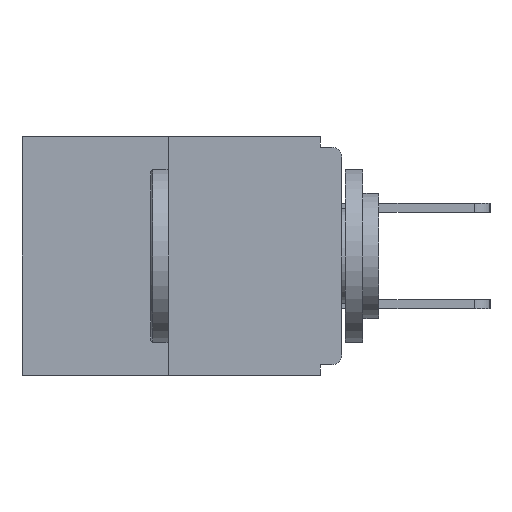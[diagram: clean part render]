
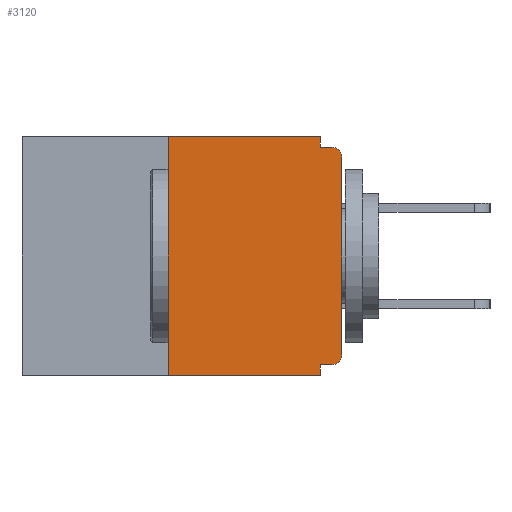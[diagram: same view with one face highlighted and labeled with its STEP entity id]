
A CAD part, left-side view. The second image highlights one B-rep face of the part: STEP entity #3120.
In plain terms, the highlighted planar face has unit normal (-1, 0, 0).
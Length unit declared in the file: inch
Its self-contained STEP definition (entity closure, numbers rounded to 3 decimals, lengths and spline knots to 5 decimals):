
#136 = DIRECTION ( 'NONE',  ( -1., 0., 0. ) ) ;
#253 = DIRECTION ( 'NONE',  ( 0., 0., -1. ) ) ;
#395 = ORIENTED_EDGE ( 'NONE', *, *, #1870, .T. ) ;
#508 = DIRECTION ( 'NONE',  ( 0., 0., 1. ) ) ;
#666 = ORIENTED_EDGE ( 'NONE', *, *, #10971, .F. ) ;
#798 = DIRECTION ( 'NONE',  ( 0., -1., 0. ) ) ;
#856 = LINE ( 'NONE', #7410, #12276 ) ;
#897 = ORIENTED_EDGE ( 'NONE', *, *, #1680, .F. ) ;
#1203 = DIRECTION ( 'NONE',  ( 0., 0., -1. ) ) ;
#1207 = VERTEX_POINT ( 'NONE', #2862 ) ;
#1286 = VERTEX_POINT ( 'NONE', #4184 ) ;
#1444 = AXIS2_PLACEMENT_3D ( 'NONE', #9204, #136, #1203 ) ;
#1544 = CARTESIAN_POINT ( 'NONE',  ( 0., 0., -0.313 ) ) ;
#1654 = LINE ( 'NONE', #8985, #3957 ) ;
#1680 = EDGE_CURVE ( 'NONE', #10077, #8715, #10153, .T. ) ;
#1840 = EDGE_CURVE ( 'NONE', #1286, #8715, #12437, .T. ) ;
#1843 = DIRECTION ( 'NONE',  ( 0., 0., 1. ) ) ;
#1870 = EDGE_CURVE ( 'NONE', #4796, #1286, #8736, .T. ) ;
#2024 = EDGE_CURVE ( 'NONE', #9354, #7687, #9660, .T. ) ;
#2215 = CARTESIAN_POINT ( 'NONE',  ( 0., 0.031, 0. ) ) ;
#2283 = EDGE_CURVE ( 'NONE', #7687, #10648, #856, .T. ) ;
#2366 = DIRECTION ( 'NONE',  ( 0., -1., 0. ) ) ;
#2507 = AXIS2_PLACEMENT_3D ( 'NONE', #6550, #2586, #12384 ) ;
#2586 = DIRECTION ( 'NONE',  ( 1., 0., 0. ) ) ;
#2814 = ORIENTED_EDGE ( 'NONE', *, *, #11748, .F. ) ;
#2862 = CARTESIAN_POINT ( 'NONE',  ( 0., 0.031, -0.343 ) ) ;
#2890 = CARTESIAN_POINT ( 'NONE',  ( 0., 0.25, 0. ) ) ;
#3120 = ADVANCED_FACE ( 'NONE', ( #11782 ), #4464, .F. ) ;
#3428 = EDGE_CURVE ( 'NONE', #9354, #1207, #8566, .T. ) ;
#3470 = EDGE_CURVE ( 'NONE', #10443, #4796, #7802, .T. ) ;
#3684 = CARTESIAN_POINT ( 'NONE',  ( 0., 0., -0.015 ) ) ;
#3781 = CARTESIAN_POINT ( 'NONE',  ( 0., 0.25, -0.343 ) ) ;
#3923 = ORIENTED_EDGE ( 'NONE', *, *, #1840, .T. ) ;
#3928 = CARTESIAN_POINT ( 'NONE',  ( 0., 0.031, -0.343 ) ) ;
#3957 = VECTOR ( 'NONE', #9028, 39.37008 ) ;
#4184 = CARTESIAN_POINT ( 'NONE',  ( 0., 0., -0.03 ) ) ;
#4430 = DIRECTION ( 'NONE',  ( 0., 0., -1. ) ) ;
#4464 = PLANE ( 'NONE',  #2507 ) ;
#4641 = EDGE_LOOP ( 'NONE', ( #4935, #12086, #10550, #8387, #666, #7011, #395, #3923, #897, #2814 ) ) ;
#4671 = CARTESIAN_POINT ( 'NONE',  ( 0., 0.031, -0.015 ) ) ;
#4796 = VERTEX_POINT ( 'NONE', #1544 ) ;
#4822 = LINE ( 'NONE', #3928, #5462 ) ;
#4935 = ORIENTED_EDGE ( 'NONE', *, *, #2283, .F. ) ;
#5242 = CARTESIAN_POINT ( 'NONE',  ( 0., 0., 0. ) ) ;
#5258 = AXIS2_PLACEMENT_3D ( 'NONE', #6522, #5469, #4430 ) ;
#5462 = VECTOR ( 'NONE', #10885, 39.37008 ) ;
#5469 = DIRECTION ( 'NONE',  ( -1., 0., 0. ) ) ;
#5792 = CARTESIAN_POINT ( 'NONE',  ( 0., 0.25, 0. ) ) ;
#6522 = CARTESIAN_POINT ( 'NONE',  ( 0., 0.015, -0.313 ) ) ;
#6541 = CARTESIAN_POINT ( 'NONE',  ( 0., 0.015, -0.328 ) ) ;
#6550 = CARTESIAN_POINT ( 'NONE',  ( 0., 0.46, 0. ) ) ;
#6869 = VECTOR ( 'NONE', #10292, 39.37008 ) ;
#7011 = ORIENTED_EDGE ( 'NONE', *, *, #3470, .T. ) ;
#7177 = CARTESIAN_POINT ( 'NONE',  ( 0., 0.031, 0. ) ) ;
#7237 = VERTEX_POINT ( 'NONE', #10142 ) ;
#7410 = CARTESIAN_POINT ( 'NONE',  ( 0., 0.46, 0. ) ) ;
#7521 = VECTOR ( 'NONE', #253, 39.37008 ) ;
#7611 = EDGE_CURVE ( 'NONE', #7237, #1207, #4822, .T. ) ;
#7687 = VERTEX_POINT ( 'NONE', #2890 ) ;
#7802 = CIRCLE ( 'NONE', #5258, 0.015 ) ;
#8295 = LINE ( 'NONE', #7177, #7521 ) ;
#8387 = ORIENTED_EDGE ( 'NONE', *, *, #7611, .F. ) ;
#8566 = LINE ( 'NONE', #11113, #6869 ) ;
#8715 = VERTEX_POINT ( 'NONE', #12147 ) ;
#8736 = LINE ( 'NONE', #5242, #11061 ) ;
#8985 = CARTESIAN_POINT ( 'NONE',  ( 0., 0., -0.328 ) ) ;
#9028 = DIRECTION ( 'NONE',  ( 0., 1., 0. ) ) ;
#9057 = VECTOR ( 'NONE', #798, 39.37008 ) ;
#9204 = CARTESIAN_POINT ( 'NONE',  ( 0., 0.015, -0.03 ) ) ;
#9354 = VERTEX_POINT ( 'NONE', #3781 ) ;
#9660 = LINE ( 'NONE', #5792, #10598 ) ;
#10077 = VERTEX_POINT ( 'NONE', #4671 ) ;
#10142 = CARTESIAN_POINT ( 'NONE',  ( 0., 0.031, -0.328 ) ) ;
#10153 = LINE ( 'NONE', #3684, #9057 ) ;
#10292 = DIRECTION ( 'NONE',  ( 0., -1., 0. ) ) ;
#10443 = VERTEX_POINT ( 'NONE', #6541 ) ;
#10550 = ORIENTED_EDGE ( 'NONE', *, *, #3428, .T. ) ;
#10598 = VECTOR ( 'NONE', #1843, 39.37008 ) ;
#10648 = VERTEX_POINT ( 'NONE', #2215 ) ;
#10885 = DIRECTION ( 'NONE',  ( 0., 0., -1. ) ) ;
#10971 = EDGE_CURVE ( 'NONE', #10443, #7237, #1654, .T. ) ;
#11061 = VECTOR ( 'NONE', #508, 39.37008 ) ;
#11113 = CARTESIAN_POINT ( 'NONE',  ( 0., 0.46, -0.343 ) ) ;
#11748 = EDGE_CURVE ( 'NONE', #10648, #10077, #8295, .T. ) ;
#11782 = FACE_OUTER_BOUND ( 'NONE', #4641, .T. ) ;
#12086 = ORIENTED_EDGE ( 'NONE', *, *, #2024, .F. ) ;
#12147 = CARTESIAN_POINT ( 'NONE',  ( 0., 0.015, -0.015 ) ) ;
#12276 = VECTOR ( 'NONE', #2366, 39.37008 ) ;
#12384 = DIRECTION ( 'NONE',  ( 0., 0., -1. ) ) ;
#12437 = CIRCLE ( 'NONE', #1444, 0.015 ) ;
